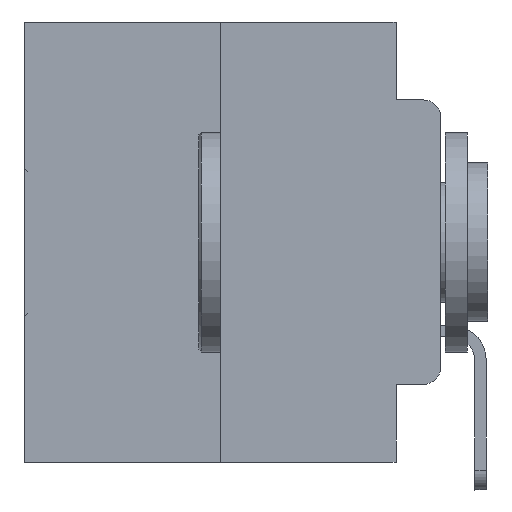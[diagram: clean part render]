
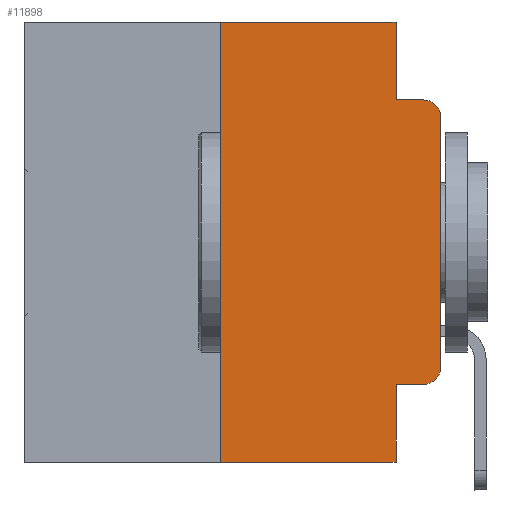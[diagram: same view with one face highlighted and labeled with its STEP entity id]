
A CAD part, left-side view. The second image highlights one B-rep face of the part: STEP entity #11898.
In plain terms, the highlighted planar face has unit normal (-1, 0, 0).
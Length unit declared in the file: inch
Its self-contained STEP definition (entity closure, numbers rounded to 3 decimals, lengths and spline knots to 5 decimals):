
#387 = CIRCLE ( 'NONE', #23221, 0.02 ) ;
#909 = ORIENTED_EDGE ( 'NONE', *, *, #5625, .T. ) ;
#1001 = CARTESIAN_POINT ( 'NONE',  ( 0., 0.02, -0.3915 ) ) ;
#1061 = CARTESIAN_POINT ( 'NONE',  ( 0., 0., -0.3915 ) ) ;
#1070 = DIRECTION ( 'NONE',  ( 0., 0., 1. ) ) ;
#2017 = DIRECTION ( 'NONE',  ( 1., 0., 0. ) ) ;
#2356 = LINE ( 'NONE', #2512, #23933 ) ;
#2512 = CARTESIAN_POINT ( 'NONE',  ( 0., 0.051, -0.0885 ) ) ;
#2546 = CARTESIAN_POINT ( 'NONE',  ( 0., 0.051, -0.4115 ) ) ;
#2998 = LINE ( 'NONE', #14916, #29539 ) ;
#3149 = VERTEX_POINT ( 'NONE', #9438 ) ;
#3235 = VERTEX_POINT ( 'NONE', #7518 ) ;
#4079 = LINE ( 'NONE', #17941, #17776 ) ;
#4091 = CARTESIAN_POINT ( 'NONE',  ( 0., 0.473, -0.5 ) ) ;
#4933 = LINE ( 'NONE', #21932, #21185 ) ;
#5086 = DIRECTION ( 'NONE',  ( -1., 0., 0. ) ) ;
#5545 = VECTOR ( 'NONE', #23465, 39.37008 ) ;
#5625 = EDGE_CURVE ( 'NONE', #16372, #7469, #4079, .T. ) ;
#5907 = CARTESIAN_POINT ( 'NONE',  ( 0., 0.051, 0. ) ) ;
#5963 = CARTESIAN_POINT ( 'NONE',  ( 0., 0.02, -0.0885 ) ) ;
#6095 = DIRECTION ( 'NONE',  ( -1., 0., 0. ) ) ;
#6470 = CARTESIAN_POINT ( 'NONE',  ( 0., 0.051, 0. ) ) ;
#6514 = VERTEX_POINT ( 'NONE', #19903 ) ;
#6802 = VERTEX_POINT ( 'NONE', #10491 ) ;
#7090 = EDGE_CURVE ( 'NONE', #6514, #25383, #2356, .T. ) ;
#7285 = VERTEX_POINT ( 'NONE', #6470 ) ;
#7465 = VECTOR ( 'NONE', #24945, 39.37008 ) ;
#7469 = VERTEX_POINT ( 'NONE', #9940 ) ;
#7518 = CARTESIAN_POINT ( 'NONE',  ( 0., 0.051, -0.4115 ) ) ;
#8629 = CARTESIAN_POINT ( 'NONE',  ( 0., 0.25, -0.5 ) ) ;
#9291 = EDGE_CURVE ( 'NONE', #3149, #16372, #23043, .T. ) ;
#9438 = CARTESIAN_POINT ( 'NONE',  ( 0., 0.02, -0.4115 ) ) ;
#9940 = CARTESIAN_POINT ( 'NONE',  ( 0., 0., -0.1085 ) ) ;
#10147 = DIRECTION ( 'NONE',  ( 0., -1., 0. ) ) ;
#10491 = CARTESIAN_POINT ( 'NONE',  ( 0., 0.051, -0.5 ) ) ;
#11367 = ORIENTED_EDGE ( 'NONE', *, *, #9291, .T. ) ;
#11765 = DIRECTION ( 'NONE',  ( 0., -1., 0. ) ) ;
#11898 = ADVANCED_FACE ( 'NONE', ( #23772 ), #24222, .F. ) ;
#12119 = LINE ( 'NONE', #21496, #28694 ) ;
#12169 = CARTESIAN_POINT ( 'NONE',  ( 0., 0.473, 0. ) ) ;
#12792 = EDGE_CURVE ( 'NONE', #29078, #7285, #2998, .T. ) ;
#13060 = EDGE_CURVE ( 'NONE', #26052, #6802, #23310, .T. ) ;
#13406 = AXIS2_PLACEMENT_3D ( 'NONE', #1001, #6095, #18030 ) ;
#14199 = EDGE_CURVE ( 'NONE', #3235, #6802, #29974, .T. ) ;
#14636 = DIRECTION ( 'NONE',  ( 0., 0., -1. ) ) ;
#14916 = CARTESIAN_POINT ( 'NONE',  ( 0., 0.473, 0. ) ) ;
#15751 = EDGE_CURVE ( 'NONE', #7469, #25383, #387, .T. ) ;
#16183 = CARTESIAN_POINT ( 'NONE',  ( 0., 0.25, 0. ) ) ;
#16372 = VERTEX_POINT ( 'NONE', #1061 ) ;
#16965 = ORIENTED_EDGE ( 'NONE', *, *, #14199, .F. ) ;
#17776 = VECTOR ( 'NONE', #1070, 39.37008 ) ;
#17941 = CARTESIAN_POINT ( 'NONE',  ( 0., 0., 0. ) ) ;
#18030 = DIRECTION ( 'NONE',  ( 0., 0., -1. ) ) ;
#19401 = ORIENTED_EDGE ( 'NONE', *, *, #26142, .F. ) ;
#19833 = DIRECTION ( 'NONE',  ( 0., -1., 0. ) ) ;
#19842 = ORIENTED_EDGE ( 'NONE', *, *, #24417, .F. ) ;
#19903 = CARTESIAN_POINT ( 'NONE',  ( 0., 0.051, -0.0885 ) ) ;
#20678 = ORIENTED_EDGE ( 'NONE', *, *, #12792, .F. ) ;
#21185 = VECTOR ( 'NONE', #14636, 39.37008 ) ;
#21496 = CARTESIAN_POINT ( 'NONE',  ( 0., 0.25, 0. ) ) ;
#21932 = CARTESIAN_POINT ( 'NONE',  ( 0., 0.051, 0. ) ) ;
#21952 = ORIENTED_EDGE ( 'NONE', *, *, #30074, .T. ) ;
#23043 = CIRCLE ( 'NONE', #13406, 0.02 ) ;
#23221 = AXIS2_PLACEMENT_3D ( 'NONE', #24283, #5086, #26806 ) ;
#23310 = LINE ( 'NONE', #4091, #5545 ) ;
#23465 = DIRECTION ( 'NONE',  ( 0., -1., 0. ) ) ;
#23772 = FACE_OUTER_BOUND ( 'NONE', #26329, .T. ) ;
#23786 = ORIENTED_EDGE ( 'NONE', *, *, #15751, .T. ) ;
#23933 = VECTOR ( 'NONE', #19833, 39.37008 ) ;
#24222 = PLANE ( 'NONE',  #30315 ) ;
#24283 = CARTESIAN_POINT ( 'NONE',  ( 0., 0.02, -0.1085 ) ) ;
#24318 = DIRECTION ( 'NONE',  ( 0., 0., 1. ) ) ;
#24417 = EDGE_CURVE ( 'NONE', #26052, #29078, #12119, .T. ) ;
#24630 = VECTOR ( 'NONE', #11765, 39.37008 ) ;
#24945 = DIRECTION ( 'NONE',  ( 0., 0., -1. ) ) ;
#25383 = VERTEX_POINT ( 'NONE', #5963 ) ;
#26052 = VERTEX_POINT ( 'NONE', #8629 ) ;
#26142 = EDGE_CURVE ( 'NONE', #7285, #6514, #4933, .T. ) ;
#26329 = EDGE_LOOP ( 'NONE', ( #909, #23786, #29792, #19401, #20678, #19842, #29217, #16965, #21952, #11367 ) ) ;
#26804 = LINE ( 'NONE', #2546, #24630 ) ;
#26806 = DIRECTION ( 'NONE',  ( 0., 0., -1. ) ) ;
#28334 = DIRECTION ( 'NONE',  ( 0., 0., -1. ) ) ;
#28694 = VECTOR ( 'NONE', #24318, 39.37008 ) ;
#29078 = VERTEX_POINT ( 'NONE', #16183 ) ;
#29217 = ORIENTED_EDGE ( 'NONE', *, *, #13060, .T. ) ;
#29539 = VECTOR ( 'NONE', #10147, 39.37008 ) ;
#29792 = ORIENTED_EDGE ( 'NONE', *, *, #7090, .F. ) ;
#29974 = LINE ( 'NONE', #5907, #7465 ) ;
#30074 = EDGE_CURVE ( 'NONE', #3235, #3149, #26804, .T. ) ;
#30315 = AXIS2_PLACEMENT_3D ( 'NONE', #12169, #2017, #28334 ) ;
